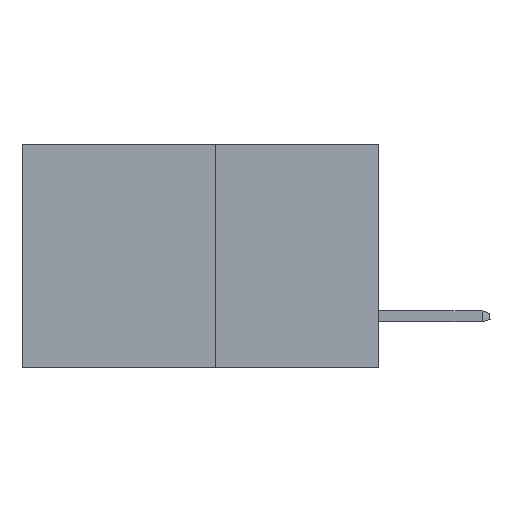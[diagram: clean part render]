
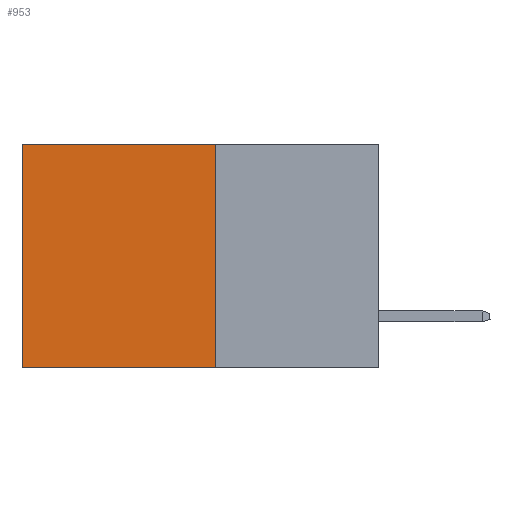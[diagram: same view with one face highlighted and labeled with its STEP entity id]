
A CAD part, left-side view. The second image highlights one B-rep face of the part: STEP entity #953.
In plain terms, the highlighted planar face has unit normal (-1, 0, 0).
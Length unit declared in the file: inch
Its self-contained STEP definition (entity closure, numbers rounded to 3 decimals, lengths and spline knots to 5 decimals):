
#145 = CARTESIAN_POINT ( 'NONE',  ( 0.277, 0.27, 0. ) ) ;
#953 = ADVANCED_FACE ( 'NONE', ( #9306 ), #13036, .F. ) ;
#1756 = EDGE_CURVE ( 'NONE', #3855, #14739, #18028, .T. ) ;
#3243 = LINE ( 'NONE', #4434, #9985 ) ;
#3306 = ORIENTED_EDGE ( 'NONE', *, *, #11144, .T. ) ;
#3855 = VERTEX_POINT ( 'NONE', #5101 ) ;
#3990 = CARTESIAN_POINT ( 'NONE',  ( 0.277, 0.27, -0.37 ) ) ;
#4434 = CARTESIAN_POINT ( 'NONE',  ( 0.277, 0.59, -0.37 ) ) ;
#4590 = VECTOR ( 'NONE', #16796, 39.37008 ) ;
#5101 = CARTESIAN_POINT ( 'NONE',  ( 0.277, 0.27, -0.37 ) ) ;
#5199 = CARTESIAN_POINT ( 'NONE',  ( 0.277, 0.27, -0.37 ) ) ;
#7299 = VECTOR ( 'NONE', #16330, 39.37008 ) ;
#8882 = LINE ( 'NONE', #3990, #4590 ) ;
#9306 = FACE_OUTER_BOUND ( 'NONE', #14999, .T. ) ;
#9500 = LINE ( 'NONE', #14833, #16520 ) ;
#9985 = VECTOR ( 'NONE', #13058, 39.37008 ) ;
#10319 = EDGE_CURVE ( 'NONE', #12340, #14739, #3243, .T. ) ;
#10322 = ORIENTED_EDGE ( 'NONE', *, *, #10319, .T. ) ;
#10911 = DIRECTION ( 'NONE',  ( 0., 0., -1. ) ) ;
#11144 = EDGE_CURVE ( 'NONE', #17560, #12340, #9500, .T. ) ;
#11880 = AXIS2_PLACEMENT_3D ( 'NONE', #16441, #12993, #10911 ) ;
#12340 = VERTEX_POINT ( 'NONE', #16393 ) ;
#12993 = DIRECTION ( 'NONE',  ( 1., 0., 0. ) ) ;
#13036 = PLANE ( 'NONE',  #11880 ) ;
#13058 = DIRECTION ( 'NONE',  ( 0., 0., -1. ) ) ;
#13517 = DIRECTION ( 'NONE',  ( 0., 1., 0. ) ) ;
#14054 = ORIENTED_EDGE ( 'NONE', *, *, #15241, .F. ) ;
#14739 = VERTEX_POINT ( 'NONE', #15064 ) ;
#14833 = CARTESIAN_POINT ( 'NONE',  ( 0.277, 0.27, 0. ) ) ;
#14999 = EDGE_LOOP ( 'NONE', ( #10322, #15245, #14054, #3306 ) ) ;
#15064 = CARTESIAN_POINT ( 'NONE',  ( 0.277, 0.59, -0.37 ) ) ;
#15241 = EDGE_CURVE ( 'NONE', #17560, #3855, #8882, .T. ) ;
#15245 = ORIENTED_EDGE ( 'NONE', *, *, #1756, .F. ) ;
#16330 = DIRECTION ( 'NONE',  ( 0., 1., 0. ) ) ;
#16393 = CARTESIAN_POINT ( 'NONE',  ( 0.277, 0.59, 0. ) ) ;
#16441 = CARTESIAN_POINT ( 'NONE',  ( 0.277, 0.27, -0.37 ) ) ;
#16520 = VECTOR ( 'NONE', #13517, 39.37008 ) ;
#16796 = DIRECTION ( 'NONE',  ( 0., 0., -1. ) ) ;
#17560 = VERTEX_POINT ( 'NONE', #145 ) ;
#18028 = LINE ( 'NONE', #5199, #7299 ) ;
